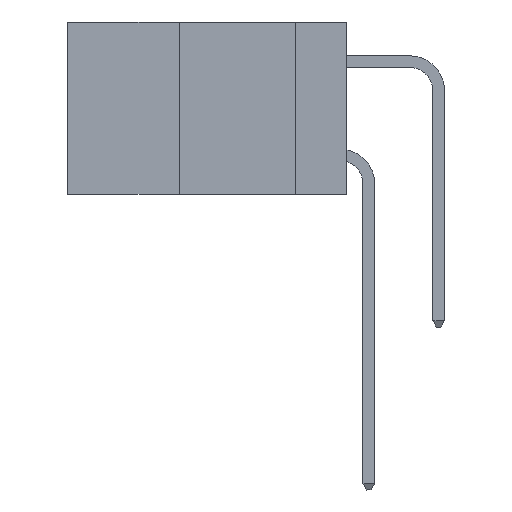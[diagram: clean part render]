
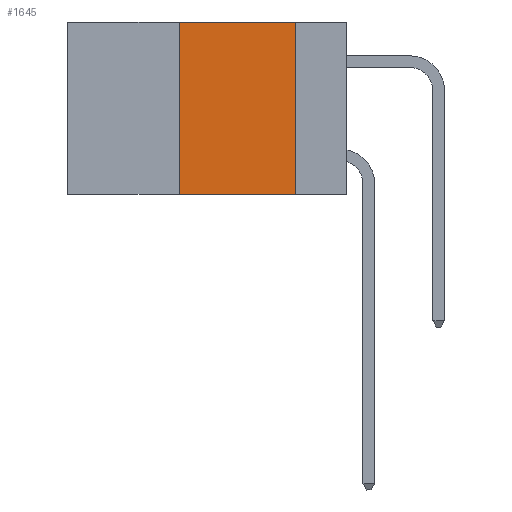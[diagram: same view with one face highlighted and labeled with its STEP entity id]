
A CAD part, left-side view. The second image highlights one B-rep face of the part: STEP entity #1645.
In plain terms, the highlighted planar face has unit normal (-1, 0, 0).
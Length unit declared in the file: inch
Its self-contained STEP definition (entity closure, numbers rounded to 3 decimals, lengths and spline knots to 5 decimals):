
#19 = CARTESIAN_POINT ( 'NONE',  ( 0., 0.11, -0.37 ) ) ;
#135 = ORIENTED_EDGE ( 'NONE', *, *, #3466, .F. ) ;
#1309 = ORIENTED_EDGE ( 'NONE', *, *, #1654, .T. ) ;
#1506 = ORIENTED_EDGE ( 'NONE', *, *, #5597, .F. ) ;
#1590 = LINE ( 'NONE', #4943, #6136 ) ;
#1645 = ADVANCED_FACE ( 'NONE', ( #5307 ), #1951, .F. ) ;
#1654 = EDGE_CURVE ( 'NONE', #8342, #5834, #3451, .T. ) ;
#1951 = PLANE ( 'NONE',  #9108 ) ;
#2281 = CARTESIAN_POINT ( 'NONE',  ( 0., 0.36, 0. ) ) ;
#2361 = EDGE_LOOP ( 'NONE', ( #135, #1506, #4129, #1309 ) ) ;
#2533 = VERTEX_POINT ( 'NONE', #9294 ) ;
#3451 = LINE ( 'NONE', #10229, #7232 ) ;
#3466 = EDGE_CURVE ( 'NONE', #2533, #5834, #5905, .T. ) ;
#3551 = VECTOR ( 'NONE', #7761, 39.37008 ) ;
#3684 = VERTEX_POINT ( 'NONE', #2281 ) ;
#4129 = ORIENTED_EDGE ( 'NONE', *, *, #9344, .F. ) ;
#4943 = CARTESIAN_POINT ( 'NONE',  ( 0., 0.6, 0. ) ) ;
#5307 = FACE_OUTER_BOUND ( 'NONE', #2361, .T. ) ;
#5354 = DIRECTION ( 'NONE',  ( 0., 0., 1. ) ) ;
#5597 = EDGE_CURVE ( 'NONE', #3684, #2533, #1590, .T. ) ;
#5834 = VERTEX_POINT ( 'NONE', #19 ) ;
#5905 = LINE ( 'NONE', #7441, #3551 ) ;
#6136 = VECTOR ( 'NONE', #7111, 39.37008 ) ;
#6265 = DIRECTION ( 'NONE',  ( 0., 0., -1. ) ) ;
#6598 = CARTESIAN_POINT ( 'NONE',  ( 0., 0.6, 0. ) ) ;
#7111 = DIRECTION ( 'NONE',  ( 0., -1., 0. ) ) ;
#7232 = VECTOR ( 'NONE', #7803, 39.37008 ) ;
#7441 = CARTESIAN_POINT ( 'NONE',  ( 0., 0.11, 0. ) ) ;
#7761 = DIRECTION ( 'NONE',  ( 0., 0., -1. ) ) ;
#7803 = DIRECTION ( 'NONE',  ( 0., -1., 0. ) ) ;
#8342 = VERTEX_POINT ( 'NONE', #11110 ) ;
#9108 = AXIS2_PLACEMENT_3D ( 'NONE', #6598, #9189, #6265 ) ;
#9189 = DIRECTION ( 'NONE',  ( 1., 0., 0. ) ) ;
#9294 = CARTESIAN_POINT ( 'NONE',  ( 0., 0.11, 0. ) ) ;
#9344 = EDGE_CURVE ( 'NONE', #8342, #3684, #10803, .T. ) ;
#10229 = CARTESIAN_POINT ( 'NONE',  ( 0., 0.6, -0.37 ) ) ;
#10268 = CARTESIAN_POINT ( 'NONE',  ( 0., 0.36, 0. ) ) ;
#10559 = VECTOR ( 'NONE', #5354, 39.37008 ) ;
#10803 = LINE ( 'NONE', #10268, #10559 ) ;
#11110 = CARTESIAN_POINT ( 'NONE',  ( 0., 0.36, -0.37 ) ) ;
